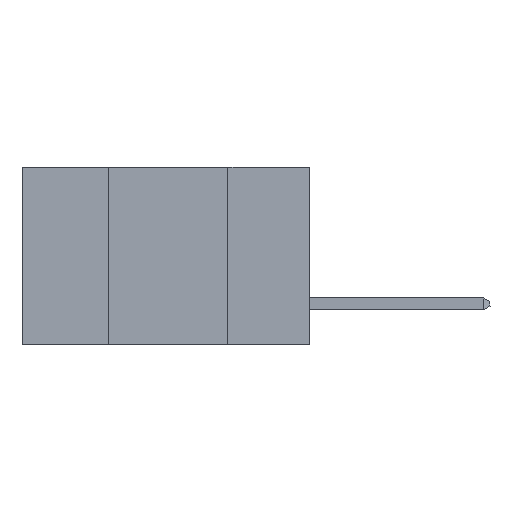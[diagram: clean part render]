
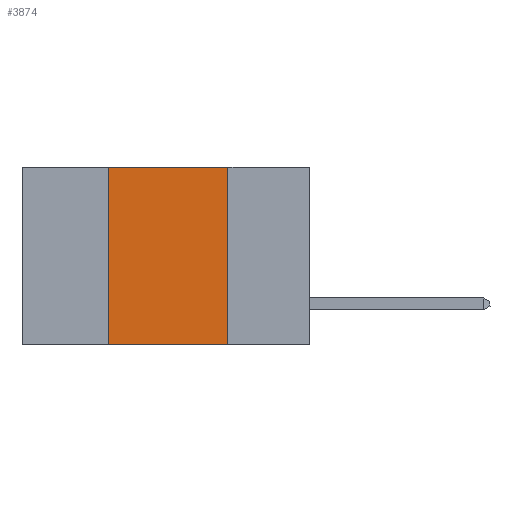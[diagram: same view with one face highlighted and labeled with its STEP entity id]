
A CAD part, left-side view. The second image highlights one B-rep face of the part: STEP entity #3874.
In plain terms, the highlighted planar face has unit normal (-1, 0, 0).
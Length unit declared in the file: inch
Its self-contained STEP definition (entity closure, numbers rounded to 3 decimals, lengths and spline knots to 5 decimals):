
#300 = LINE ( 'NONE', #19120, #4306 ) ;
#1423 = AXIS2_PLACEMENT_3D ( 'NONE', #8418, #15175, #5097 ) ;
#1682 = VECTOR ( 'NONE', #21743, 39.37008 ) ;
#1786 = EDGE_CURVE ( 'NONE', #9941, #18702, #7159, .T. ) ;
#2201 = LINE ( 'NONE', #4949, #1682 ) ;
#2684 = VECTOR ( 'NONE', #20438, 39.37008 ) ;
#3338 = CARTESIAN_POINT ( 'NONE',  ( 0., 0.42, 0. ) ) ;
#3874 = ADVANCED_FACE ( 'NONE', ( #15742 ), #13455, .F. ) ;
#4306 = VECTOR ( 'NONE', #20779, 39.37008 ) ;
#4891 = EDGE_LOOP ( 'NONE', ( #15360, #13247, #20877, #20589 ) ) ;
#4949 = CARTESIAN_POINT ( 'NONE',  ( 0., 0.6, 0. ) ) ;
#5097 = DIRECTION ( 'NONE',  ( 0., 0., -1. ) ) ;
#6721 = DIRECTION ( 'NONE',  ( 0., 0., 1. ) ) ;
#6734 = EDGE_CURVE ( 'NONE', #16401, #9028, #2201, .T. ) ;
#7021 = EDGE_CURVE ( 'NONE', #9028, #18702, #300, .T. ) ;
#7159 = LINE ( 'NONE', #10371, #2684 ) ;
#7400 = CARTESIAN_POINT ( 'NONE',  ( 0., 0.17, -0.37 ) ) ;
#8418 = CARTESIAN_POINT ( 'NONE',  ( 0., 0.6, 0. ) ) ;
#8570 = EDGE_CURVE ( 'NONE', #9941, #16401, #13427, .T. ) ;
#9028 = VERTEX_POINT ( 'NONE', #16326 ) ;
#9941 = VERTEX_POINT ( 'NONE', #19124 ) ;
#10039 = CARTESIAN_POINT ( 'NONE',  ( 0., 0.42, 0. ) ) ;
#10371 = CARTESIAN_POINT ( 'NONE',  ( 0., 0.6, -0.37 ) ) ;
#13247 = ORIENTED_EDGE ( 'NONE', *, *, #6734, .F. ) ;
#13427 = LINE ( 'NONE', #3338, #16120 ) ;
#13455 = PLANE ( 'NONE',  #1423 ) ;
#15175 = DIRECTION ( 'NONE',  ( 1., 0., 0. ) ) ;
#15360 = ORIENTED_EDGE ( 'NONE', *, *, #7021, .F. ) ;
#15742 = FACE_OUTER_BOUND ( 'NONE', #4891, .T. ) ;
#16120 = VECTOR ( 'NONE', #6721, 39.37008 ) ;
#16326 = CARTESIAN_POINT ( 'NONE',  ( 0., 0.17, 0. ) ) ;
#16401 = VERTEX_POINT ( 'NONE', #10039 ) ;
#18702 = VERTEX_POINT ( 'NONE', #7400 ) ;
#19120 = CARTESIAN_POINT ( 'NONE',  ( 0., 0.17, 0. ) ) ;
#19124 = CARTESIAN_POINT ( 'NONE',  ( 0., 0.42, -0.37 ) ) ;
#20438 = DIRECTION ( 'NONE',  ( 0., -1., 0. ) ) ;
#20589 = ORIENTED_EDGE ( 'NONE', *, *, #1786, .T. ) ;
#20779 = DIRECTION ( 'NONE',  ( 0., 0., -1. ) ) ;
#20877 = ORIENTED_EDGE ( 'NONE', *, *, #8570, .F. ) ;
#21743 = DIRECTION ( 'NONE',  ( 0., -1., 0. ) ) ;
